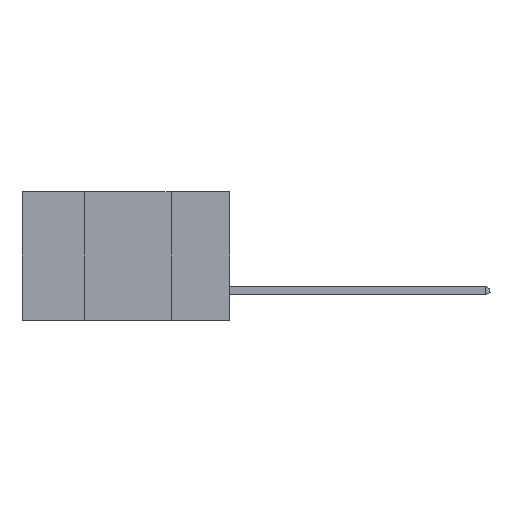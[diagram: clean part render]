
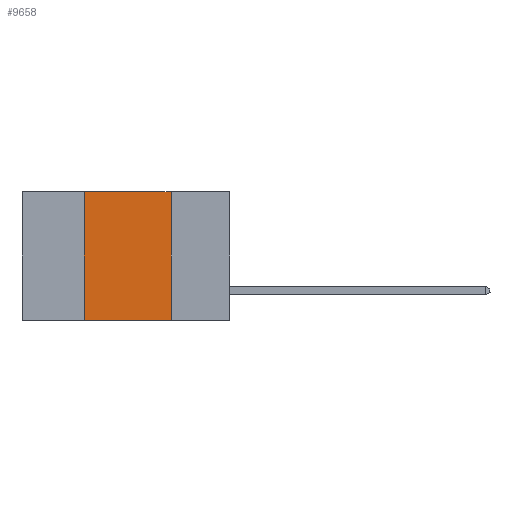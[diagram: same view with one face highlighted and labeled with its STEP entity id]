
A CAD part, left-side view. The second image highlights one B-rep face of the part: STEP entity #9658.
In plain terms, the highlighted planar face has unit normal (-1, 0, 0).
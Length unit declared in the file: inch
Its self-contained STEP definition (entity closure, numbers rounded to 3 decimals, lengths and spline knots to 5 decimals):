
#1572 = EDGE_CURVE ( 'NONE', #12283, #5326, #10185, .T. ) ;
#1612 = DIRECTION ( 'NONE',  ( 0., -1., 0. ) ) ;
#1730 = VECTOR ( 'NONE', #12477, 39.37008 ) ;
#2329 = VERTEX_POINT ( 'NONE', #10546 ) ;
#2334 = DIRECTION ( 'NONE',  ( 0., 0., -1. ) ) ;
#3754 = VECTOR ( 'NONE', #5561, 39.37008 ) ;
#4511 = LINE ( 'NONE', #12185, #3754 ) ;
#4586 = DIRECTION ( 'NONE',  ( 1., 0., 0. ) ) ;
#4945 = AXIS2_PLACEMENT_3D ( 'NONE', #12896, #4586, #12964 ) ;
#5326 = VERTEX_POINT ( 'NONE', #7889 ) ;
#5513 = VECTOR ( 'NONE', #1612, 39.37008 ) ;
#5561 = DIRECTION ( 'NONE',  ( 0., -1., 0. ) ) ;
#5638 = EDGE_LOOP ( 'NONE', ( #12016, #15931, #13886, #10031 ) ) ;
#5827 = CARTESIAN_POINT ( 'NONE',  ( 0., 0.42, -0.37 ) ) ;
#7773 = EDGE_CURVE ( 'NONE', #12283, #2329, #12929, .T. ) ;
#7889 = CARTESIAN_POINT ( 'NONE',  ( 0., 0.17, -0.37 ) ) ;
#9030 = FACE_OUTER_BOUND ( 'NONE', #5638, .T. ) ;
#9075 = CARTESIAN_POINT ( 'NONE',  ( 0., 0.42, 0. ) ) ;
#9658 = ADVANCED_FACE ( 'NONE', ( #9030 ), #16292, .F. ) ;
#10031 = ORIENTED_EDGE ( 'NONE', *, *, #1572, .T. ) ;
#10185 = LINE ( 'NONE', #18323, #5513 ) ;
#10546 = CARTESIAN_POINT ( 'NONE',  ( 0., 0.42, 0. ) ) ;
#12016 = ORIENTED_EDGE ( 'NONE', *, *, #15187, .F. ) ;
#12185 = CARTESIAN_POINT ( 'NONE',  ( 0., 0.6, 0. ) ) ;
#12283 = VERTEX_POINT ( 'NONE', #5827 ) ;
#12477 = DIRECTION ( 'NONE',  ( 0., 0., 1. ) ) ;
#12896 = CARTESIAN_POINT ( 'NONE',  ( 0., 0.6, 0. ) ) ;
#12929 = LINE ( 'NONE', #9075, #1730 ) ;
#12964 = DIRECTION ( 'NONE',  ( 0., 0., -1. ) ) ;
#13886 = ORIENTED_EDGE ( 'NONE', *, *, #7773, .F. ) ;
#14962 = EDGE_CURVE ( 'NONE', #2329, #19600, #4511, .T. ) ;
#15187 = EDGE_CURVE ( 'NONE', #19600, #5326, #19315, .T. ) ;
#15853 = CARTESIAN_POINT ( 'NONE',  ( 0., 0.17, 0. ) ) ;
#15931 = ORIENTED_EDGE ( 'NONE', *, *, #14962, .F. ) ;
#16292 = PLANE ( 'NONE',  #4945 ) ;
#18323 = CARTESIAN_POINT ( 'NONE',  ( 0., 0.6, -0.37 ) ) ;
#19047 = CARTESIAN_POINT ( 'NONE',  ( 0., 0.17, 0. ) ) ;
#19315 = LINE ( 'NONE', #15853, #20366 ) ;
#19600 = VERTEX_POINT ( 'NONE', #19047 ) ;
#20366 = VECTOR ( 'NONE', #2334, 39.37008 ) ;
